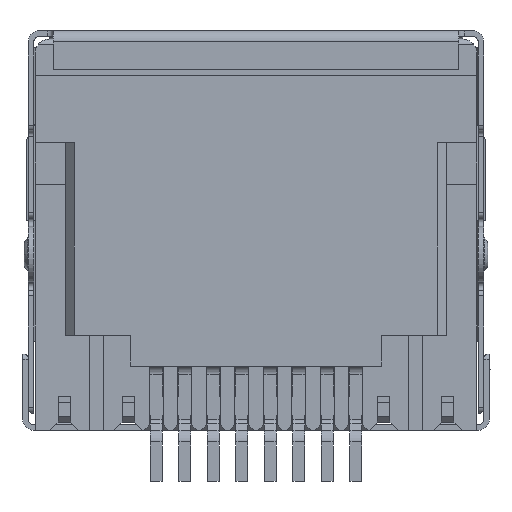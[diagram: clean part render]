
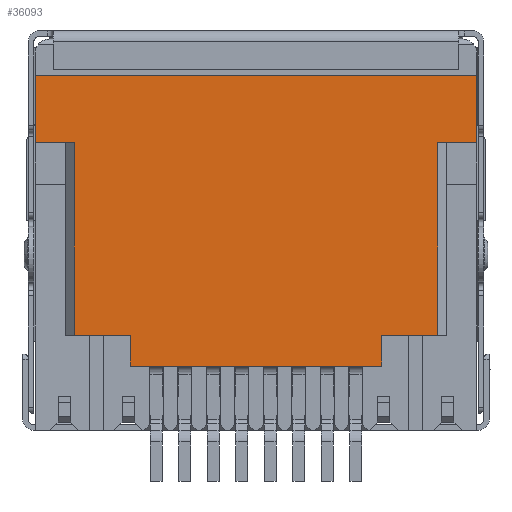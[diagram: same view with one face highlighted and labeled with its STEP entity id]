
A CAD part, front view. The second image highlights one B-rep face of the part: STEP entity #36093.
In plain terms, the highlighted planar face has unit normal (0, -1, 0).
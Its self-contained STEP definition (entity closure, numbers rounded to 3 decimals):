
#311 = FACE_OUTER_BOUND ( 'NONE', #11630, .T. ) ;
#1336 = EDGE_CURVE ( 'NONE', #2543, #32601, #23606, .T. ) ;
#1958 = VECTOR ( 'NONE', #4660, 1000. ) ;
#2543 = VERTEX_POINT ( 'NONE', #21480 ) ;
#3444 = CARTESIAN_POINT ( 'NONE',  ( -6.5, -5.525, -3.7 ) ) ;
#3747 = VERTEX_POINT ( 'NONE', #32095 ) ;
#3887 = CARTESIAN_POINT ( 'NONE',  ( 4.5, -5.525, -11.7 ) ) ;
#4660 = DIRECTION ( 'NONE',  ( 1., 0., 0. ) ) ;
#4856 = VERTEX_POINT ( 'NONE', #11205 ) ;
#4883 = VECTOR ( 'NONE', #19031, 1000. ) ;
#5783 = VECTOR ( 'NONE', #22208, 1000. ) ;
#5927 = EDGE_CURVE ( 'NONE', #6987, #28962, #19756, .T. ) ;
#6658 = ORIENTED_EDGE ( 'NONE', *, *, #19361, .T. ) ;
#6987 = VERTEX_POINT ( 'NONE', #11757 ) ;
#7659 = DIRECTION ( 'NONE',  ( 0., 0., -1. ) ) ;
#7916 = ORIENTED_EDGE ( 'NONE', *, *, #5927, .T. ) ;
#7971 = VECTOR ( 'NONE', #41425, 1000. ) ;
#8825 = LINE ( 'NONE', #13474, #25067 ) ;
#10323 = CARTESIAN_POINT ( 'NONE',  ( 7.9, -5.525, -3.7 ) ) ;
#11003 = CARTESIAN_POINT ( 'NONE',  ( -7.9, -5.525, -10.6 ) ) ;
#11205 = CARTESIAN_POINT ( 'NONE',  ( 6.5, -5.525, -3.7 ) ) ;
#11630 = EDGE_LOOP ( 'NONE', ( #27315, #40291, #29872, #41975, #7916, #36957, #31157, #17457, #6658, #13751, #34341, #13342 ) ) ;
#11757 = CARTESIAN_POINT ( 'NONE',  ( -7.9, -5.525, -3.7 ) ) ;
#12033 = LINE ( 'NONE', #12993, #20122 ) ;
#12292 = PLANE ( 'NONE',  #22354 ) ;
#12488 = LINE ( 'NONE', #34867, #29275 ) ;
#12993 = CARTESIAN_POINT ( 'NONE',  ( -7.9, -5.525, -10.6 ) ) ;
#13203 = LINE ( 'NONE', #15108, #14372 ) ;
#13207 = VECTOR ( 'NONE', #14308, 1000. ) ;
#13342 = ORIENTED_EDGE ( 'NONE', *, *, #30900, .T. ) ;
#13474 = CARTESIAN_POINT ( 'NONE',  ( 6.5, -5.525, -14. ) ) ;
#13751 = ORIENTED_EDGE ( 'NONE', *, *, #38045, .T. ) ;
#14308 = DIRECTION ( 'NONE',  ( 0., 0., -1. ) ) ;
#14372 = VECTOR ( 'NONE', #7659, 1000. ) ;
#15108 = CARTESIAN_POINT ( 'NONE',  ( -4.5, -5.525, -10.6 ) ) ;
#15861 = DIRECTION ( 'NONE',  ( 0., 0., -1. ) ) ;
#16843 = DIRECTION ( 'NONE',  ( -1., 0., 0. ) ) ;
#17035 = DIRECTION ( 'NONE',  ( 0., 0., 1. ) ) ;
#17457 = ORIENTED_EDGE ( 'NONE', *, *, #33906, .T. ) ;
#18846 = DIRECTION ( 'NONE',  ( 0., 0., 1. ) ) ;
#19031 = DIRECTION ( 'NONE',  ( 0., 0., 1. ) ) ;
#19200 = CARTESIAN_POINT ( 'NONE',  ( -7.9, -5.525, -14. ) ) ;
#19361 = EDGE_CURVE ( 'NONE', #3747, #28080, #21337, .T. ) ;
#19625 = VERTEX_POINT ( 'NONE', #43014 ) ;
#19756 = LINE ( 'NONE', #45446, #46446 ) ;
#20122 = VECTOR ( 'NONE', #36026, 1000. ) ;
#21337 = LINE ( 'NONE', #41578, #7971 ) ;
#21480 = CARTESIAN_POINT ( 'NONE',  ( 7.9, -5.525, -1.3 ) ) ;
#21576 = LINE ( 'NONE', #29873, #34361 ) ;
#22208 = DIRECTION ( 'NONE',  ( 1., 0., 0. ) ) ;
#22354 = AXIS2_PLACEMENT_3D ( 'NONE', #26873, #41688, #15861 ) ;
#22918 = EDGE_CURVE ( 'NONE', #31799, #31638, #40047, .T. ) ;
#23111 = CARTESIAN_POINT ( 'NONE',  ( -7.9, -5.525, -3.7 ) ) ;
#23606 = LINE ( 'NONE', #40750, #29979 ) ;
#23940 = EDGE_CURVE ( 'NONE', #28962, #33107, #25978, .T. ) ;
#25067 = VECTOR ( 'NONE', #17035, 1000. ) ;
#25978 = LINE ( 'NONE', #29235, #13207 ) ;
#26193 = EDGE_CURVE ( 'NONE', #6987, #38939, #30410, .T. ) ;
#26873 = CARTESIAN_POINT ( 'NONE',  ( -7.9, -5.525, -14. ) ) ;
#27315 = ORIENTED_EDGE ( 'NONE', *, *, #37442, .T. ) ;
#27532 = EDGE_CURVE ( 'NONE', #33107, #19625, #12033, .T. ) ;
#28080 = VERTEX_POINT ( 'NONE', #3887 ) ;
#28962 = VERTEX_POINT ( 'NONE', #3444 ) ;
#29235 = CARTESIAN_POINT ( 'NONE',  ( -6.5, -5.525, -14. ) ) ;
#29275 = VECTOR ( 'NONE', #16843, 1000. ) ;
#29677 = DIRECTION ( 'NONE',  ( 0., 0., -1. ) ) ;
#29872 = ORIENTED_EDGE ( 'NONE', *, *, #35644, .T. ) ;
#29873 = CARTESIAN_POINT ( 'NONE',  ( 4.5, -5.525, -10.6 ) ) ;
#29979 = VECTOR ( 'NONE', #29677, 1000. ) ;
#30325 = DIRECTION ( 'NONE',  ( 1., 0., 0. ) ) ;
#30365 = LINE ( 'NONE', #23111, #1958 ) ;
#30410 = LINE ( 'NONE', #19200, #4883 ) ;
#30900 = EDGE_CURVE ( 'NONE', #31638, #4856, #8825, .T. ) ;
#31157 = ORIENTED_EDGE ( 'NONE', *, *, #27532, .T. ) ;
#31170 = CARTESIAN_POINT ( 'NONE',  ( 4.5, -5.525, -10.6 ) ) ;
#31638 = VERTEX_POINT ( 'NONE', #47346 ) ;
#31799 = VERTEX_POINT ( 'NONE', #31170 ) ;
#32095 = CARTESIAN_POINT ( 'NONE',  ( -4.5, -5.525, -11.7 ) ) ;
#32601 = VERTEX_POINT ( 'NONE', #10323 ) ;
#33107 = VERTEX_POINT ( 'NONE', #39671 ) ;
#33906 = EDGE_CURVE ( 'NONE', #19625, #3747, #13203, .T. ) ;
#34341 = ORIENTED_EDGE ( 'NONE', *, *, #22918, .T. ) ;
#34361 = VECTOR ( 'NONE', #18846, 1000. ) ;
#34867 = CARTESIAN_POINT ( 'NONE',  ( -7.9, -5.525, -1.3 ) ) ;
#35644 = EDGE_CURVE ( 'NONE', #2543, #38939, #12488, .T. ) ;
#36026 = DIRECTION ( 'NONE',  ( 1., 0., 0. ) ) ;
#36093 = ADVANCED_FACE ( 'NONE', ( #311 ), #12292, .T. ) ;
#36957 = ORIENTED_EDGE ( 'NONE', *, *, #23940, .T. ) ;
#37442 = EDGE_CURVE ( 'NONE', #4856, #32601, #30365, .T. ) ;
#38045 = EDGE_CURVE ( 'NONE', #28080, #31799, #21576, .T. ) ;
#38939 = VERTEX_POINT ( 'NONE', #46683 ) ;
#39671 = CARTESIAN_POINT ( 'NONE',  ( -6.5, -5.525, -10.6 ) ) ;
#40047 = LINE ( 'NONE', #11003, #5783 ) ;
#40291 = ORIENTED_EDGE ( 'NONE', *, *, #1336, .F. ) ;
#40750 = CARTESIAN_POINT ( 'NONE',  ( 7.9, -5.525, -14. ) ) ;
#41425 = DIRECTION ( 'NONE',  ( 1., 0., 0. ) ) ;
#41578 = CARTESIAN_POINT ( 'NONE',  ( -7.9, -5.525, -11.7 ) ) ;
#41688 = DIRECTION ( 'NONE',  ( 0., -1., 0. ) ) ;
#41975 = ORIENTED_EDGE ( 'NONE', *, *, #26193, .F. ) ;
#43014 = CARTESIAN_POINT ( 'NONE',  ( -4.5, -5.525, -10.6 ) ) ;
#45446 = CARTESIAN_POINT ( 'NONE',  ( -7.9, -5.525, -3.7 ) ) ;
#46446 = VECTOR ( 'NONE', #30325, 1000. ) ;
#46683 = CARTESIAN_POINT ( 'NONE',  ( -7.9, -5.525, -1.3 ) ) ;
#47346 = CARTESIAN_POINT ( 'NONE',  ( 6.5, -5.525, -10.6 ) ) ;
